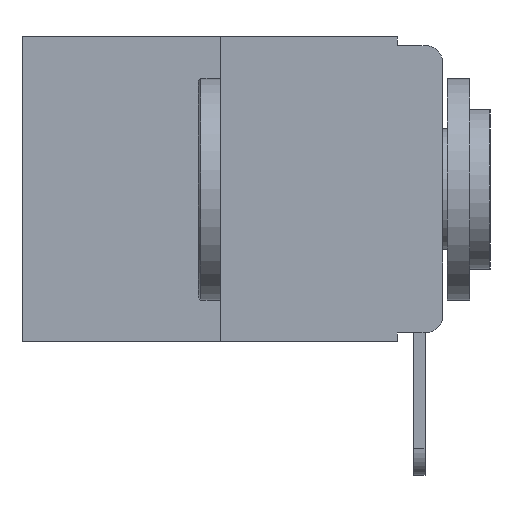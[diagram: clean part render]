
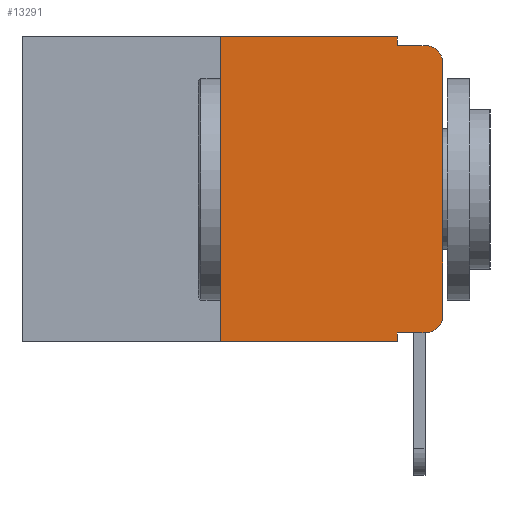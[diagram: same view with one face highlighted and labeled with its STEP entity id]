
A CAD part, left-side view. The second image highlights one B-rep face of the part: STEP entity #13291.
In plain terms, the highlighted planar face has unit normal (-1, 0, 0).
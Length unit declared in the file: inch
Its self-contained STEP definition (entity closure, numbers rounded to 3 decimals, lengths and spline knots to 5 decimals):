
#387 = CARTESIAN_POINT ( 'NONE',  ( 0., 0.473, 0. ) ) ;
#898 = EDGE_CURVE ( 'NONE', #6514, #17443, #14288, .T. ) ;
#1151 = DIRECTION ( 'NONE',  ( 0., -1., 0. ) ) ;
#1390 = EDGE_CURVE ( 'NONE', #4030, #2095, #13347, .T. ) ;
#1754 = VECTOR ( 'NONE', #1151, 39.37008 ) ;
#1868 = CARTESIAN_POINT ( 'NONE',  ( 0., 0.02, -0.01 ) ) ;
#1872 = DIRECTION ( 'NONE',  ( 0., -1., 0. ) ) ;
#1912 = EDGE_CURVE ( 'NONE', #12828, #15431, #16416, .T. ) ;
#2095 = VERTEX_POINT ( 'NONE', #2107 ) ;
#2107 = CARTESIAN_POINT ( 'NONE',  ( 0., 0., -0.03 ) ) ;
#2439 = VECTOR ( 'NONE', #11670, 39.37008 ) ;
#2515 = ORIENTED_EDGE ( 'NONE', *, *, #14658, .T. ) ;
#2625 = DIRECTION ( 'NONE',  ( 0., 0., 1. ) ) ;
#2752 = EDGE_CURVE ( 'NONE', #7255, #11598, #21864, .T. ) ;
#2824 = CARTESIAN_POINT ( 'NONE',  ( 0., 0.051, -0.01 ) ) ;
#2937 = CARTESIAN_POINT ( 'NONE',  ( 0., 0.051, -0.01 ) ) ;
#3064 = EDGE_CURVE ( 'NONE', #17443, #15359, #11195, .T. ) ;
#3486 = VECTOR ( 'NONE', #4780, 39.37008 ) ;
#3490 = DIRECTION ( 'NONE',  ( 0., 0., -1. ) ) ;
#3957 = VECTOR ( 'NONE', #1872, 39.37008 ) ;
#4030 = VERTEX_POINT ( 'NONE', #6055 ) ;
#4347 = ORIENTED_EDGE ( 'NONE', *, *, #3064, .F. ) ;
#4551 = ORIENTED_EDGE ( 'NONE', *, *, #2752, .F. ) ;
#4766 = ORIENTED_EDGE ( 'NONE', *, *, #10090, .T. ) ;
#4780 = DIRECTION ( 'NONE',  ( 0., 0., -1. ) ) ;
#4860 = ORIENTED_EDGE ( 'NONE', *, *, #8408, .T. ) ;
#4903 = DIRECTION ( 'NONE',  ( -1., 0., 0. ) ) ;
#5055 = DIRECTION ( 'NONE',  ( 0., 0., -1. ) ) ;
#5428 = ORIENTED_EDGE ( 'NONE', *, *, #1390, .T. ) ;
#5990 = CARTESIAN_POINT ( 'NONE',  ( 0., 0.473, 0. ) ) ;
#6055 = CARTESIAN_POINT ( 'NONE',  ( 0., 0., -0.313 ) ) ;
#6514 = VERTEX_POINT ( 'NONE', #16137 ) ;
#7255 = VERTEX_POINT ( 'NONE', #2824 ) ;
#8019 = DIRECTION ( 'NONE',  ( 0., -1., 0. ) ) ;
#8408 = EDGE_CURVE ( 'NONE', #12828, #11956, #8729, .T. ) ;
#8483 = DIRECTION ( 'NONE',  ( -1., 0., 0. ) ) ;
#8729 = LINE ( 'NONE', #17041, #3957 ) ;
#9104 = ORIENTED_EDGE ( 'NONE', *, *, #1912, .F. ) ;
#9156 = VECTOR ( 'NONE', #2625, 39.37008 ) ;
#9273 = ORIENTED_EDGE ( 'NONE', *, *, #18560, .F. ) ;
#9478 = CARTESIAN_POINT ( 'NONE',  ( 0., 0.051, -0.343 ) ) ;
#9685 = CARTESIAN_POINT ( 'NONE',  ( 0., 0.02, -0.03 ) ) ;
#9801 = CARTESIAN_POINT ( 'NONE',  ( 0., 0.02, -0.333 ) ) ;
#10090 = EDGE_CURVE ( 'NONE', #11956, #4030, #16692, .T. ) ;
#10524 = EDGE_LOOP ( 'NONE', ( #5428, #2515, #4551, #9273, #4347, #18050, #12292, #9104, #4860, #4766 ) ) ;
#10941 = VECTOR ( 'NONE', #8019, 39.37008 ) ;
#11195 = LINE ( 'NONE', #5990, #19789 ) ;
#11598 = VERTEX_POINT ( 'NONE', #1868 ) ;
#11670 = DIRECTION ( 'NONE',  ( 0., 0., 1. ) ) ;
#11846 = CARTESIAN_POINT ( 'NONE',  ( 0., 0.051, -0.333 ) ) ;
#11956 = VERTEX_POINT ( 'NONE', #9801 ) ;
#12254 = CARTESIAN_POINT ( 'NONE',  ( 0., 0.02, -0.313 ) ) ;
#12292 = ORIENTED_EDGE ( 'NONE', *, *, #13450, .T. ) ;
#12495 = CARTESIAN_POINT ( 'NONE',  ( 0., 0.25, 0. ) ) ;
#12558 = CARTESIAN_POINT ( 'NONE',  ( 0., 0.25, 0. ) ) ;
#12828 = VERTEX_POINT ( 'NONE', #11846 ) ;
#12932 = CARTESIAN_POINT ( 'NONE',  ( 0., 0.051, 0. ) ) ;
#13236 = DIRECTION ( 'NONE',  ( 0., 0., -1. ) ) ;
#13291 = ADVANCED_FACE ( 'NONE', ( #15137 ), #21878, .F. ) ;
#13347 = LINE ( 'NONE', #20072, #2439 ) ;
#13438 = VECTOR ( 'NONE', #5055, 39.37008 ) ;
#13450 = EDGE_CURVE ( 'NONE', #6514, #15431, #14893, .T. ) ;
#14288 = LINE ( 'NONE', #12495, #9156 ) ;
#14658 = EDGE_CURVE ( 'NONE', #2095, #11598, #17707, .T. ) ;
#14893 = LINE ( 'NONE', #16639, #1754 ) ;
#15033 = LINE ( 'NONE', #15134, #13438 ) ;
#15134 = CARTESIAN_POINT ( 'NONE',  ( 0., 0.051, 0. ) ) ;
#15137 = FACE_OUTER_BOUND ( 'NONE', #10524, .T. ) ;
#15359 = VERTEX_POINT ( 'NONE', #12932 ) ;
#15431 = VERTEX_POINT ( 'NONE', #9478 ) ;
#15533 = AXIS2_PLACEMENT_3D ( 'NONE', #387, #17128, #3490 ) ;
#16137 = CARTESIAN_POINT ( 'NONE',  ( 0., 0.25, -0.343 ) ) ;
#16416 = LINE ( 'NONE', #20042, #3486 ) ;
#16639 = CARTESIAN_POINT ( 'NONE',  ( 0., 0.473, -0.343 ) ) ;
#16692 = CIRCLE ( 'NONE', #19513, 0.02 ) ;
#17041 = CARTESIAN_POINT ( 'NONE',  ( 0., 0.051, -0.333 ) ) ;
#17128 = DIRECTION ( 'NONE',  ( 1., 0., 0. ) ) ;
#17227 = DIRECTION ( 'NONE',  ( 0., 0., -1. ) ) ;
#17443 = VERTEX_POINT ( 'NONE', #12558 ) ;
#17707 = CIRCLE ( 'NONE', #21244, 0.02 ) ;
#18050 = ORIENTED_EDGE ( 'NONE', *, *, #898, .F. ) ;
#18560 = EDGE_CURVE ( 'NONE', #15359, #7255, #15033, .T. ) ;
#19513 = AXIS2_PLACEMENT_3D ( 'NONE', #12254, #8483, #17227 ) ;
#19789 = VECTOR ( 'NONE', #21391, 39.37008 ) ;
#20042 = CARTESIAN_POINT ( 'NONE',  ( 0., 0.051, 0. ) ) ;
#20072 = CARTESIAN_POINT ( 'NONE',  ( 0., 0., 0. ) ) ;
#21244 = AXIS2_PLACEMENT_3D ( 'NONE', #9685, #4903, #13236 ) ;
#21391 = DIRECTION ( 'NONE',  ( 0., -1., 0. ) ) ;
#21864 = LINE ( 'NONE', #2937, #10941 ) ;
#21878 = PLANE ( 'NONE',  #15533 ) ;
